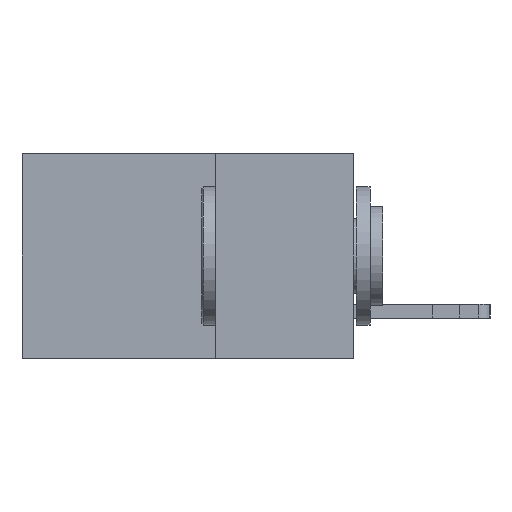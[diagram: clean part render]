
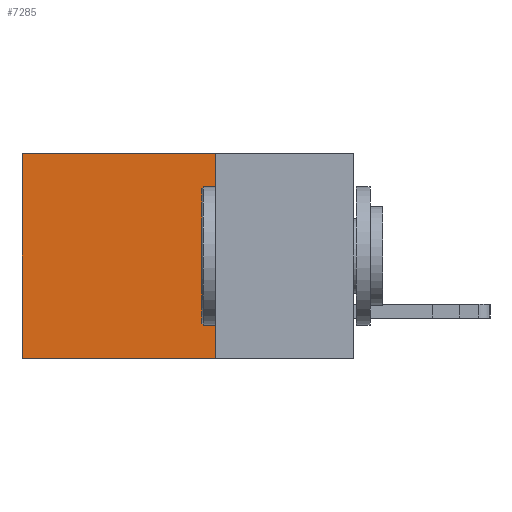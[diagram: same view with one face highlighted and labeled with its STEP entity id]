
A CAD part, left-side view. The second image highlights one B-rep face of the part: STEP entity #7285.
In plain terms, the highlighted planar face has unit normal (-1, 0, 0).
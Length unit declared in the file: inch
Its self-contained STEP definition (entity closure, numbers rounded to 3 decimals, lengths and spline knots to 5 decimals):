
#433 = ORIENTED_EDGE ( 'NONE', *, *, #3473, .T. ) ;
#582 = LINE ( 'NONE', #9226, #4272 ) ;
#1805 = CARTESIAN_POINT ( 'NONE',  ( 0.2875, 0.6, -0.37 ) ) ;
#2334 = CARTESIAN_POINT ( 'NONE',  ( 0.2875, 0.25, 0. ) ) ;
#2513 = LINE ( 'NONE', #2334, #8678 ) ;
#3193 = EDGE_LOOP ( 'NONE', ( #9159, #17188, #9928, #433 ) ) ;
#3473 = EDGE_CURVE ( 'NONE', #16581, #8586, #2513, .T. ) ;
#3485 = DIRECTION ( 'NONE',  ( 0., 0., -1. ) ) ;
#4272 = VECTOR ( 'NONE', #10234, 39.37008 ) ;
#5322 = VECTOR ( 'NONE', #3485, 39.37008 ) ;
#5569 = CARTESIAN_POINT ( 'NONE',  ( 0.2875, 0.25, -0.37 ) ) ;
#5723 = CARTESIAN_POINT ( 'NONE',  ( 0.2875, 0.25, -0.37 ) ) ;
#6457 = CARTESIAN_POINT ( 'NONE',  ( 0.2875, 0.6, 0. ) ) ;
#6721 = PLANE ( 'NONE',  #9347 ) ;
#7285 = ADVANCED_FACE ( 'NONE', ( #8182 ), #6721, .F. ) ;
#8167 = VERTEX_POINT ( 'NONE', #1805 ) ;
#8182 = FACE_OUTER_BOUND ( 'NONE', #3193, .T. ) ;
#8586 = VERTEX_POINT ( 'NONE', #6457 ) ;
#8592 = DIRECTION ( 'NONE',  ( 0., 1., 0. ) ) ;
#8678 = VECTOR ( 'NONE', #11237, 39.37008 ) ;
#9070 = EDGE_CURVE ( 'NONE', #17198, #8167, #9778, .T. ) ;
#9159 = ORIENTED_EDGE ( 'NONE', *, *, #16343, .T. ) ;
#9226 = CARTESIAN_POINT ( 'NONE',  ( 0.2875, 0.6, 0. ) ) ;
#9347 = AXIS2_PLACEMENT_3D ( 'NONE', #17457, #16172, #16083 ) ;
#9778 = LINE ( 'NONE', #5569, #15513 ) ;
#9928 = ORIENTED_EDGE ( 'NONE', *, *, #10609, .F. ) ;
#10234 = DIRECTION ( 'NONE',  ( 0., 0., -1. ) ) ;
#10609 = EDGE_CURVE ( 'NONE', #16581, #17198, #12967, .T. ) ;
#11237 = DIRECTION ( 'NONE',  ( 0., 1., 0. ) ) ;
#12967 = LINE ( 'NONE', #13058, #5322 ) ;
#13058 = CARTESIAN_POINT ( 'NONE',  ( 0.2875, 0.25, 0. ) ) ;
#15513 = VECTOR ( 'NONE', #8592, 39.37008 ) ;
#16083 = DIRECTION ( 'NONE',  ( 0., 0., -1. ) ) ;
#16172 = DIRECTION ( 'NONE',  ( 1., 0., 0. ) ) ;
#16343 = EDGE_CURVE ( 'NONE', #8586, #8167, #582, .T. ) ;
#16581 = VERTEX_POINT ( 'NONE', #16933 ) ;
#16933 = CARTESIAN_POINT ( 'NONE',  ( 0.2875, 0.25, 0. ) ) ;
#17188 = ORIENTED_EDGE ( 'NONE', *, *, #9070, .F. ) ;
#17198 = VERTEX_POINT ( 'NONE', #5723 ) ;
#17457 = CARTESIAN_POINT ( 'NONE',  ( 0.2875, 0.25, 0. ) ) ;
